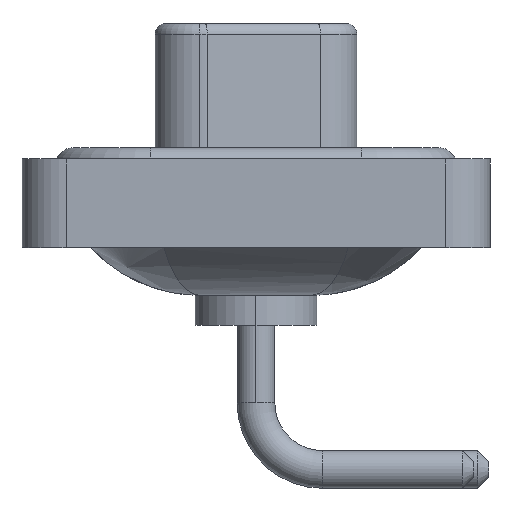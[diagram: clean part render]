
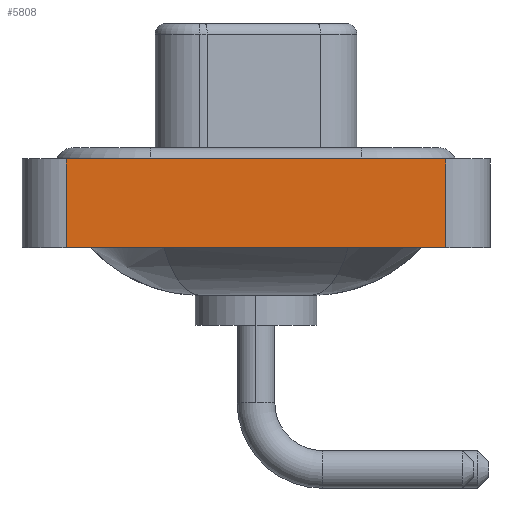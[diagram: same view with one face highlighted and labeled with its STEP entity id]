
A CAD part, left-side view. The second image highlights one B-rep face of the part: STEP entity #5808.
In plain terms, the highlighted planar face has unit normal (-1, 0, 0).
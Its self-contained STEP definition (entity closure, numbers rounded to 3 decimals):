
#57 = DIRECTION ( 'NONE',  ( 0., 0., 1. ) ) ;
#1435 = EDGE_CURVE ( 'NONE', #1995, #15731, #3006, .T. ) ;
#1995 = VERTEX_POINT ( 'NONE', #10568 ) ;
#2289 = ORIENTED_EDGE ( 'NONE', *, *, #13430, .T. ) ;
#2410 = VERTEX_POINT ( 'NONE', #7892 ) ;
#2654 = EDGE_LOOP ( 'NONE', ( #13366, #19188, #6105, #2289 ) ) ;
#3006 = LINE ( 'NONE', #13393, #7028 ) ;
#5022 = CARTESIAN_POINT ( 'NONE',  ( -7.3, -8.55, 0.4 ) ) ;
#5808 = ADVANCED_FACE ( 'NONE', ( #15030 ), #7655, .T. ) ;
#6105 = ORIENTED_EDGE ( 'NONE', *, *, #17412, .F. ) ;
#7028 = VECTOR ( 'NONE', #57, 1000. ) ;
#7478 = EDGE_CURVE ( 'NONE', #10632, #15731, #8015, .T. ) ;
#7619 = AXIS2_PLACEMENT_3D ( 'NONE', #18550, #7839, #10958 ) ;
#7655 = PLANE ( 'NONE',  #7619 ) ;
#7839 = DIRECTION ( 'NONE',  ( -1., 0., 0. ) ) ;
#7892 = CARTESIAN_POINT ( 'NONE',  ( -7.3, 8.55, -3.6 ) ) ;
#8015 = LINE ( 'NONE', #15512, #8294 ) ;
#8294 = VECTOR ( 'NONE', #9782, 1000. ) ;
#9272 = VECTOR ( 'NONE', #18622, 1000. ) ;
#9782 = DIRECTION ( 'NONE',  ( 0., -1., 0. ) ) ;
#10568 = CARTESIAN_POINT ( 'NONE',  ( -7.3, -8.55, -3.6 ) ) ;
#10632 = VERTEX_POINT ( 'NONE', #14572 ) ;
#10958 = DIRECTION ( 'NONE',  ( 0., 0., 1. ) ) ;
#11353 = VECTOR ( 'NONE', #16172, 1000. ) ;
#11697 = CARTESIAN_POINT ( 'NONE',  ( -7.3, -8.55, -3.6 ) ) ;
#12582 = CARTESIAN_POINT ( 'NONE',  ( -7.3, 8.55, -3.6 ) ) ;
#13366 = ORIENTED_EDGE ( 'NONE', *, *, #1435, .T. ) ;
#13393 = CARTESIAN_POINT ( 'NONE',  ( -7.3, -8.55, -3.6 ) ) ;
#13430 = EDGE_CURVE ( 'NONE', #2410, #1995, #19089, .T. ) ;
#14572 = CARTESIAN_POINT ( 'NONE',  ( -7.3, 8.55, 0.4 ) ) ;
#15030 = FACE_OUTER_BOUND ( 'NONE', #2654, .T. ) ;
#15512 = CARTESIAN_POINT ( 'NONE',  ( -7.3, -8.55, 0.4 ) ) ;
#15731 = VERTEX_POINT ( 'NONE', #5022 ) ;
#16172 = DIRECTION ( 'NONE',  ( 0., -1., 0. ) ) ;
#17057 = LINE ( 'NONE', #12582, #9272 ) ;
#17412 = EDGE_CURVE ( 'NONE', #2410, #10632, #17057, .T. ) ;
#18550 = CARTESIAN_POINT ( 'NONE',  ( -7.3, -8.55, -3.6 ) ) ;
#18622 = DIRECTION ( 'NONE',  ( 0., 0., 1. ) ) ;
#19089 = LINE ( 'NONE', #11697, #11353 ) ;
#19188 = ORIENTED_EDGE ( 'NONE', *, *, #7478, .F. ) ;
